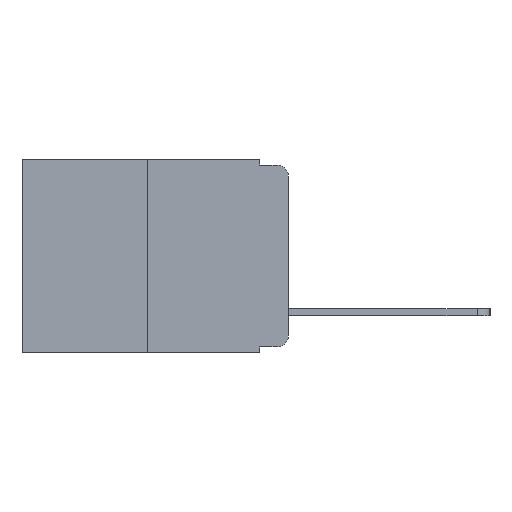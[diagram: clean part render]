
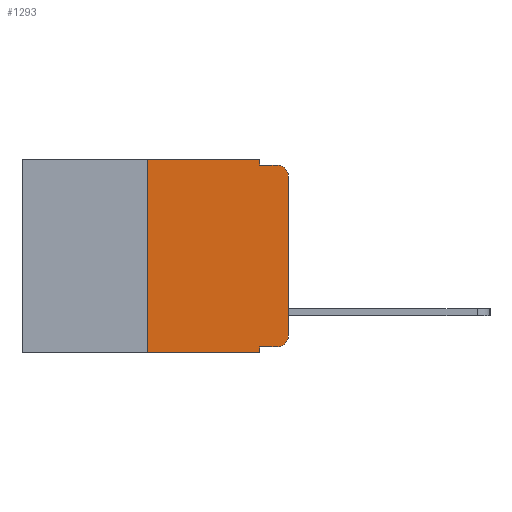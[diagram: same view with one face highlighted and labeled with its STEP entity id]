
A CAD part, left-side view. The second image highlights one B-rep face of the part: STEP entity #1293.
In plain terms, the highlighted planar face has unit normal (-1, 0, 0).
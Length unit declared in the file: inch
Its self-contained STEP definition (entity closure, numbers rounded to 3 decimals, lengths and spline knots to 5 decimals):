
#388 = LINE ( 'NONE', #5132, #7988 ) ;
#416 = DIRECTION ( 'NONE',  ( 0., -1., 0. ) ) ;
#531 = VERTEX_POINT ( 'NONE', #3585 ) ;
#806 = LINE ( 'NONE', #9015, #5130 ) ;
#928 = CARTESIAN_POINT ( 'NONE',  ( 0., 0.051, 0. ) ) ;
#936 = CARTESIAN_POINT ( 'NONE',  ( 0., 0.051, -0.343 ) ) ;
#999 = CARTESIAN_POINT ( 'NONE',  ( 0., 0., -0.03 ) ) ;
#1293 = ADVANCED_FACE ( 'NONE', ( #5890 ), #8192, .F. ) ;
#1469 = VERTEX_POINT ( 'NONE', #7148 ) ;
#1641 = LINE ( 'NONE', #928, #10536 ) ;
#2086 = VERTEX_POINT ( 'NONE', #999 ) ;
#2217 = VERTEX_POINT ( 'NONE', #6690 ) ;
#2424 = CARTESIAN_POINT ( 'NONE',  ( 0., 0.02, -0.03 ) ) ;
#2449 = CARTESIAN_POINT ( 'NONE',  ( 0., 0.051, -0.333 ) ) ;
#2543 = VECTOR ( 'NONE', #8425, 39.37008 ) ;
#2606 = CARTESIAN_POINT ( 'NONE',  ( 0., 0.25, 0. ) ) ;
#2654 = LINE ( 'NONE', #3638, #11691 ) ;
#2726 = AXIS2_PLACEMENT_3D ( 'NONE', #4874, #11045, #5760 ) ;
#2754 = AXIS2_PLACEMENT_3D ( 'NONE', #9909, #7896, #8104 ) ;
#2872 = EDGE_CURVE ( 'NONE', #4079, #9595, #1641, .T. ) ;
#3168 = VERTEX_POINT ( 'NONE', #5251 ) ;
#3190 = EDGE_CURVE ( 'NONE', #2086, #10974, #10409, .T. ) ;
#3434 = DIRECTION ( 'NONE',  ( 0., 0., -1. ) ) ;
#3555 = ORIENTED_EDGE ( 'NONE', *, *, #6554, .T. ) ;
#3585 = CARTESIAN_POINT ( 'NONE',  ( 0., 0., -0.313 ) ) ;
#3594 = DIRECTION ( 'NONE',  ( 0., -1., 0. ) ) ;
#3600 = DIRECTION ( 'NONE',  ( 0., 0., 1. ) ) ;
#3638 = CARTESIAN_POINT ( 'NONE',  ( 0., 0.473, -0.343 ) ) ;
#3898 = DIRECTION ( 'NONE',  ( 0., 0., -1. ) ) ;
#4079 = VERTEX_POINT ( 'NONE', #10636 ) ;
#4081 = EDGE_CURVE ( 'NONE', #3168, #1469, #11101, .T. ) ;
#4777 = ORIENTED_EDGE ( 'NONE', *, *, #8239, .F. ) ;
#4874 = CARTESIAN_POINT ( 'NONE',  ( 0., 0.02, -0.313 ) ) ;
#5051 = ORIENTED_EDGE ( 'NONE', *, *, #10166, .F. ) ;
#5130 = VECTOR ( 'NONE', #3594, 39.37008 ) ;
#5132 = CARTESIAN_POINT ( 'NONE',  ( 0., 0.473, 0. ) ) ;
#5251 = CARTESIAN_POINT ( 'NONE',  ( 0., 0.051, -0.333 ) ) ;
#5391 = LINE ( 'NONE', #11057, #2543 ) ;
#5397 = LINE ( 'NONE', #2606, #7486 ) ;
#5487 = EDGE_CURVE ( 'NONE', #9595, #10974, #806, .T. ) ;
#5500 = CARTESIAN_POINT ( 'NONE',  ( 0., 0.051, -0.01 ) ) ;
#5610 = ORIENTED_EDGE ( 'NONE', *, *, #8497, .T. ) ;
#5664 = CARTESIAN_POINT ( 'NONE',  ( 0., 0.02, -0.01 ) ) ;
#5760 = DIRECTION ( 'NONE',  ( 0., 0., -1. ) ) ;
#5774 = VECTOR ( 'NONE', #9457, 39.37008 ) ;
#5890 = FACE_OUTER_BOUND ( 'NONE', #6382, .T. ) ;
#6049 = LINE ( 'NONE', #8583, #5774 ) ;
#6314 = ORIENTED_EDGE ( 'NONE', *, *, #5487, .F. ) ;
#6327 = VERTEX_POINT ( 'NONE', #8184 ) ;
#6382 = EDGE_LOOP ( 'NONE', ( #3555, #8397, #6314, #6880, #4777, #5051, #5610, #10315, #10856, #11136 ) ) ;
#6554 = EDGE_CURVE ( 'NONE', #531, #2086, #5391, .T. ) ;
#6690 = CARTESIAN_POINT ( 'NONE',  ( 0., 0.25, 0. ) ) ;
#6880 = ORIENTED_EDGE ( 'NONE', *, *, #2872, .F. ) ;
#7142 = EDGE_CURVE ( 'NONE', #1469, #531, #11297, .T. ) ;
#7148 = CARTESIAN_POINT ( 'NONE',  ( 0., 0.02, -0.333 ) ) ;
#7486 = VECTOR ( 'NONE', #3600, 39.37008 ) ;
#7896 = DIRECTION ( 'NONE',  ( 1., 0., 0. ) ) ;
#7988 = VECTOR ( 'NONE', #11306, 39.37008 ) ;
#8104 = DIRECTION ( 'NONE',  ( 0., 0., -1. ) ) ;
#8184 = CARTESIAN_POINT ( 'NONE',  ( 0., 0.25, -0.343 ) ) ;
#8192 = PLANE ( 'NONE',  #2754 ) ;
#8197 = DIRECTION ( 'NONE',  ( 0., -1., 0. ) ) ;
#8239 = EDGE_CURVE ( 'NONE', #2217, #4079, #388, .T. ) ;
#8397 = ORIENTED_EDGE ( 'NONE', *, *, #3190, .T. ) ;
#8425 = DIRECTION ( 'NONE',  ( 0., 0., 1. ) ) ;
#8497 = EDGE_CURVE ( 'NONE', #6327, #11065, #2654, .T. ) ;
#8583 = CARTESIAN_POINT ( 'NONE',  ( 0., 0.051, 0. ) ) ;
#8784 = VECTOR ( 'NONE', #416, 39.37008 ) ;
#8875 = DIRECTION ( 'NONE',  ( -1., 0., 0. ) ) ;
#9015 = CARTESIAN_POINT ( 'NONE',  ( 0., 0.051, -0.01 ) ) ;
#9457 = DIRECTION ( 'NONE',  ( 0., 0., -1. ) ) ;
#9595 = VERTEX_POINT ( 'NONE', #5500 ) ;
#9909 = CARTESIAN_POINT ( 'NONE',  ( 0., 0.473, 0. ) ) ;
#10166 = EDGE_CURVE ( 'NONE', #6327, #2217, #5397, .T. ) ;
#10315 = ORIENTED_EDGE ( 'NONE', *, *, #11706, .F. ) ;
#10409 = CIRCLE ( 'NONE', #11628, 0.02 ) ;
#10536 = VECTOR ( 'NONE', #3898, 39.37008 ) ;
#10636 = CARTESIAN_POINT ( 'NONE',  ( 0., 0.051, 0. ) ) ;
#10856 = ORIENTED_EDGE ( 'NONE', *, *, #4081, .T. ) ;
#10974 = VERTEX_POINT ( 'NONE', #5664 ) ;
#11045 = DIRECTION ( 'NONE',  ( -1., 0., 0. ) ) ;
#11057 = CARTESIAN_POINT ( 'NONE',  ( 0., 0., 0. ) ) ;
#11065 = VERTEX_POINT ( 'NONE', #936 ) ;
#11101 = LINE ( 'NONE', #2449, #8784 ) ;
#11136 = ORIENTED_EDGE ( 'NONE', *, *, #7142, .T. ) ;
#11297 = CIRCLE ( 'NONE', #2726, 0.02 ) ;
#11306 = DIRECTION ( 'NONE',  ( 0., -1., 0. ) ) ;
#11628 = AXIS2_PLACEMENT_3D ( 'NONE', #2424, #8875, #3434 ) ;
#11691 = VECTOR ( 'NONE', #8197, 39.37008 ) ;
#11706 = EDGE_CURVE ( 'NONE', #3168, #11065, #6049, .T. ) ;
